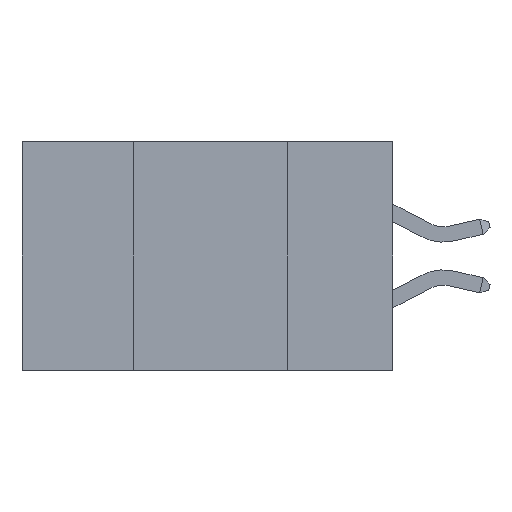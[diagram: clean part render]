
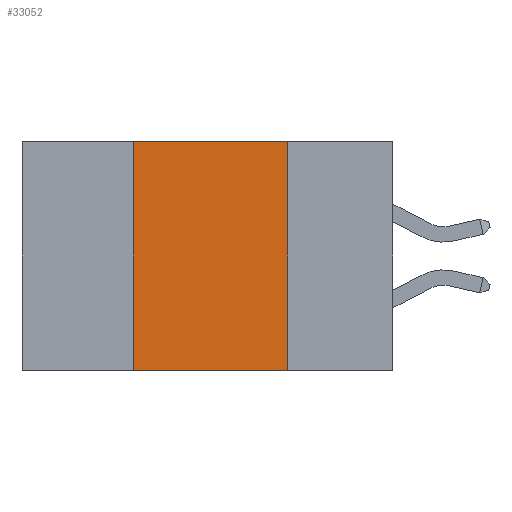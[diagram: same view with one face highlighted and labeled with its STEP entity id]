
A CAD part, left-side view. The second image highlights one B-rep face of the part: STEP entity #33052.
In plain terms, the highlighted planar face has unit normal (-1, 0, 0).
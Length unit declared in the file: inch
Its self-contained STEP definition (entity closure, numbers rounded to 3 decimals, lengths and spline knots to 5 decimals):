
#744 = VERTEX_POINT ( 'NONE', #28593 ) ;
#1308 = VECTOR ( 'NONE', #30123, 39.37008 ) ;
#2492 = CARTESIAN_POINT ( 'NONE',  ( 0., 0.6, 0. ) ) ;
#2755 = DIRECTION ( 'NONE',  ( 1., 0., 0. ) ) ;
#5283 = CARTESIAN_POINT ( 'NONE',  ( 0., 0.6, 0. ) ) ;
#7060 = EDGE_CURVE ( 'NONE', #39374, #744, #26251, .T. ) ;
#7421 = EDGE_CURVE ( 'NONE', #26054, #27874, #26710, .T. ) ;
#11181 = LINE ( 'NONE', #5283, #15267 ) ;
#11463 = DIRECTION ( 'NONE',  ( 0., -1., 0. ) ) ;
#11842 = ORIENTED_EDGE ( 'NONE', *, *, #7060, .F. ) ;
#12069 = CARTESIAN_POINT ( 'NONE',  ( 0., 0.42, 0. ) ) ;
#14535 = AXIS2_PLACEMENT_3D ( 'NONE', #2492, #2755, #31666 ) ;
#15267 = VECTOR ( 'NONE', #11463, 39.37008 ) ;
#18161 = VECTOR ( 'NONE', #41361, 39.37008 ) ;
#18691 = CARTESIAN_POINT ( 'NONE',  ( 0., 0.42, 0. ) ) ;
#21107 = FACE_OUTER_BOUND ( 'NONE', #21641, .T. ) ;
#21641 = EDGE_LOOP ( 'NONE', ( #11842, #22438, #35491, #25886 ) ) ;
#22438 = ORIENTED_EDGE ( 'NONE', *, *, #39103, .F. ) ;
#25823 = CARTESIAN_POINT ( 'NONE',  ( 0., 0.17, 0. ) ) ;
#25886 = ORIENTED_EDGE ( 'NONE', *, *, #27180, .T. ) ;
#26054 = VERTEX_POINT ( 'NONE', #32333 ) ;
#26251 = LINE ( 'NONE', #25823, #36202 ) ;
#26710 = LINE ( 'NONE', #18691, #18161 ) ;
#26756 = DIRECTION ( 'NONE',  ( 0., 0., -1. ) ) ;
#27180 = EDGE_CURVE ( 'NONE', #26054, #744, #36082, .T. ) ;
#27874 = VERTEX_POINT ( 'NONE', #12069 ) ;
#28593 = CARTESIAN_POINT ( 'NONE',  ( 0., 0.17, -0.37 ) ) ;
#30123 = DIRECTION ( 'NONE',  ( 0., -1., 0. ) ) ;
#31666 = DIRECTION ( 'NONE',  ( 0., 0., -1. ) ) ;
#32074 = PLANE ( 'NONE',  #14535 ) ;
#32333 = CARTESIAN_POINT ( 'NONE',  ( 0., 0.42, -0.37 ) ) ;
#33052 = ADVANCED_FACE ( 'NONE', ( #21107 ), #32074, .F. ) ;
#35491 = ORIENTED_EDGE ( 'NONE', *, *, #7421, .F. ) ;
#36082 = LINE ( 'NONE', #36541, #1308 ) ;
#36202 = VECTOR ( 'NONE', #26756, 39.37008 ) ;
#36541 = CARTESIAN_POINT ( 'NONE',  ( 0., 0.6, -0.37 ) ) ;
#39103 = EDGE_CURVE ( 'NONE', #27874, #39374, #11181, .T. ) ;
#39374 = VERTEX_POINT ( 'NONE', #41479 ) ;
#41361 = DIRECTION ( 'NONE',  ( 0., 0., 1. ) ) ;
#41479 = CARTESIAN_POINT ( 'NONE',  ( 0., 0.17, 0. ) ) ;
